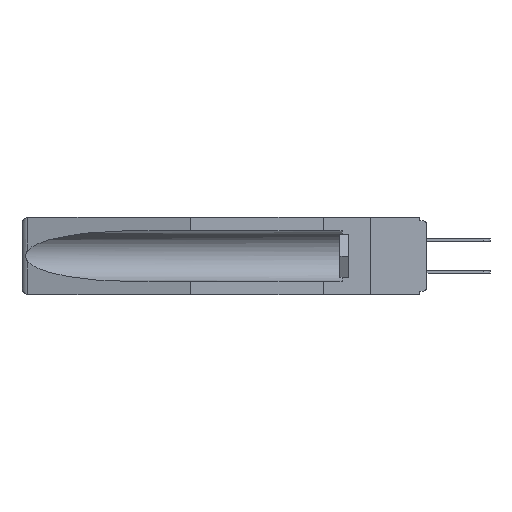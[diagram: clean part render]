
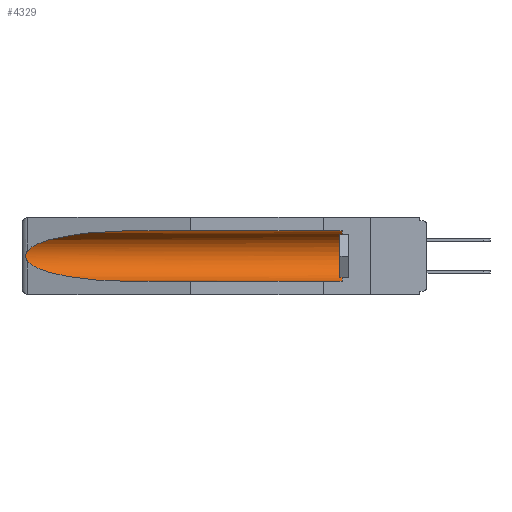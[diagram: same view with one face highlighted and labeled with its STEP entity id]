
A CAD part, left-side view. The second image highlights one B-rep face of the part: STEP entity #4329.
In plain terms, the highlighted cylindrical face has radius 2.857 mm (diameter 5.715 mm), a partial arc.
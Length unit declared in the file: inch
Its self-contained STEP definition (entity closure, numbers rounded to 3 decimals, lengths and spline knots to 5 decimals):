
#585 = DIRECTION ( 'NONE',  ( 0., 0., 1. ) ) ;
#1095 = DIRECTION ( 'NONE',  ( 0., 0., 1. ) ) ;
#1178 = CARTESIAN_POINT ( 'NONE',  ( 0.25451, 1.48313, -0.09465 ) ) ;
#1548 = EDGE_CURVE ( 'NONE', #8477, #19671, #4572, .T. ) ;
#2380 =( BOUNDED_CURVE ( )  B_SPLINE_CURVE ( 3, ( #19207, #9756, #20937, #3091 ),
 .UNSPECIFIED., .F., .F. ) 
 B_SPLINE_CURVE_WITH_KNOTS ( ( 4, 4 ),
 ( 0.1948, 1.5708 ),
 .UNSPECIFIED. ) 
 CURVE ( )  GEOMETRIC_REPRESENTATION_ITEM ( )  RATIONAL_B_SPLINE_CURVE ( ( 1., 0.848, 0.848, 1. ) ) 
 REPRESENTATION_ITEM ( '' )  );
#2488 = VERTEX_POINT ( 'NONE', #17750 ) ;
#2782 = CARTESIAN_POINT ( 'NONE',  ( 0.26597, 1.52961, -0.15275 ) ) ;
#2795 = VECTOR ( 'NONE', #6259, 39.37008 ) ;
#3091 = CARTESIAN_POINT ( 'NONE',  ( 0.155, 1.07973, -0.284 ) ) ;
#4329 = ADVANCED_FACE ( 'NONE', ( #4805 ), #20082, .F. ) ;
#4429 = CARTESIAN_POINT ( 'NONE',  ( 0.2673, 1.5327, -0.16383 ) ) ;
#4442 = ORIENTED_EDGE ( 'NONE', *, *, #8272, .T. ) ;
#4572 = LINE ( 'NONE', #4695, #2795 ) ;
#4640 = CARTESIAN_POINT ( 'NONE',  ( 0.26654, 1.53092, -0.15636 ) ) ;
#4695 = CARTESIAN_POINT ( 'NONE',  ( 0.155, -0.30754, -0.059 ) ) ;
#4805 = FACE_OUTER_BOUND ( 'NONE', #16945, .T. ) ;
#5417 = CARTESIAN_POINT ( 'NONE',  ( 0.155, -0.30754, -0.284 ) ) ;
#6072 = CARTESIAN_POINT ( 'NONE',  ( 0.26537, 1.52718, -0.19328 ) ) ;
#6249 = VERTEX_POINT ( 'NONE', #10771 ) ;
#6259 = DIRECTION ( 'NONE',  ( 0., 1., 0. ) ) ;
#6285 = CARTESIAN_POINT ( 'NONE',  ( 0.26597, 1.5296, -0.19026 ) ) ;
#6444 = CARTESIAN_POINT ( 'NONE',  ( 0.155, 1.07973, -0.059 ) ) ;
#6823 = B_SPLINE_CURVE_WITH_KNOTS ( 'NONE', 3,
 ( #12874, #2782, #4640, #4429, #16057, #14362, #15851, #7789, #6285, #6072 ),
 .UNSPECIFIED., .F., .F.,
 ( 4, 2, 2, 2, 4 ),
 ( 0., 0.00029, 0.00058, 0.00087, 0.00117 ),
 .UNSPECIFIED. ) ;
#7789 = CARTESIAN_POINT ( 'NONE',  ( 0.26655, 1.53094, -0.18657 ) ) ;
#8272 = EDGE_CURVE ( 'NONE', #15408, #6249, #6823, .T. ) ;
#8328 = ORIENTED_EDGE ( 'NONE', *, *, #1548, .T. ) ;
#8477 = VERTEX_POINT ( 'NONE', #8809 ) ;
#8479 = ORIENTED_EDGE ( 'NONE', *, *, #19051, .T. ) ;
#8809 = CARTESIAN_POINT ( 'NONE',  ( 0.155, 0.126, -0.059 ) ) ;
#9168 = ORIENTED_EDGE ( 'NONE', *, *, #12138, .T. ) ;
#9251 = CARTESIAN_POINT ( 'NONE',  ( 0.155, 0.126, -0.1715 ) ) ;
#9665 = VECTOR ( 'NONE', #15278, 39.37008 ) ;
#9756 = CARTESIAN_POINT ( 'NONE',  ( 0.25451, 1.48313, -0.24835 ) ) ;
#9853 = ORIENTED_EDGE ( 'NONE', *, *, #11145, .F. ) ;
#10570 = CARTESIAN_POINT ( 'NONE',  ( 0.155, -0.30754, -0.1715 ) ) ;
#10771 = CARTESIAN_POINT ( 'NONE',  ( 0.26537, 1.52718, -0.19328 ) ) ;
#10986 = CARTESIAN_POINT ( 'NONE',  ( 0.155, 1.07973, -0.059 ) ) ;
#11145 = EDGE_CURVE ( 'NONE', #2488, #16005, #14017, .T. ) ;
#11362 = CARTESIAN_POINT ( 'NONE',  ( 0.155, 1.07973, -0.284 ) ) ;
#11669 = CIRCLE ( 'NONE', #16961, 0.1125 ) ;
#12138 = EDGE_CURVE ( 'NONE', #2488, #8477, #11669, .T. ) ;
#12337 = DIRECTION ( 'NONE',  ( 0., -1., 0. ) ) ;
#12454 = CARTESIAN_POINT ( 'NONE',  ( 0.26537, 1.52718, -0.14972 ) ) ;
#12626 = CARTESIAN_POINT ( 'NONE',  ( 0.26537, 1.52718, -0.14972 ) ) ;
#12874 = CARTESIAN_POINT ( 'NONE',  ( 0.26537, 1.52718, -0.14972 ) ) ;
#14017 = LINE ( 'NONE', #5417, #9665 ) ;
#14362 = CARTESIAN_POINT ( 'NONE',  ( 0.2675, 1.53308, -0.17534 ) ) ;
#15278 = DIRECTION ( 'NONE',  ( 0., 1., 0. ) ) ;
#15408 = VERTEX_POINT ( 'NONE', #12454 ) ;
#15662 = EDGE_CURVE ( 'NONE', #19671, #15408, #17806, .T. ) ;
#15851 = CARTESIAN_POINT ( 'NONE',  ( 0.2673, 1.53269, -0.17917 ) ) ;
#16005 = VERTEX_POINT ( 'NONE', #11362 ) ;
#16057 = CARTESIAN_POINT ( 'NONE',  ( 0.2675, 1.53308, -0.16763 ) ) ;
#16135 = AXIS2_PLACEMENT_3D ( 'NONE', #10570, #18465, #585 ) ;
#16574 = ORIENTED_EDGE ( 'NONE', *, *, #15662, .T. ) ;
#16945 = EDGE_LOOP ( 'NONE', ( #16574, #4442, #8479, #9853, #9168, #8328 ) ) ;
#16961 = AXIS2_PLACEMENT_3D ( 'NONE', #9251, #12337, #1095 ) ;
#17750 = CARTESIAN_POINT ( 'NONE',  ( 0.155, 0.126, -0.284 ) ) ;
#17806 =( BOUNDED_CURVE ( )  B_SPLINE_CURVE ( 3, ( #10986, #18884, #1178, #12626 ),
 .UNSPECIFIED., .F., .F. ) 
 B_SPLINE_CURVE_WITH_KNOTS ( ( 4, 4 ),
 ( 4.71239, 6.08839 ),
 .UNSPECIFIED. ) 
 CURVE ( )  GEOMETRIC_REPRESENTATION_ITEM ( )  RATIONAL_B_SPLINE_CURVE ( ( 1., 0.848, 0.848, 1. ) ) 
 REPRESENTATION_ITEM ( '' )  );
#18465 = DIRECTION ( 'NONE',  ( 0., 1., 0. ) ) ;
#18884 = CARTESIAN_POINT ( 'NONE',  ( 0.21114, 1.30732, -0.059 ) ) ;
#19051 = EDGE_CURVE ( 'NONE', #6249, #16005, #2380, .T. ) ;
#19207 = CARTESIAN_POINT ( 'NONE',  ( 0.26537, 1.52718, -0.19328 ) ) ;
#19671 = VERTEX_POINT ( 'NONE', #6444 ) ;
#20082 = CYLINDRICAL_SURFACE ( 'NONE', #16135, 0.1125 ) ;
#20937 = CARTESIAN_POINT ( 'NONE',  ( 0.21114, 1.30732, -0.284 ) ) ;
